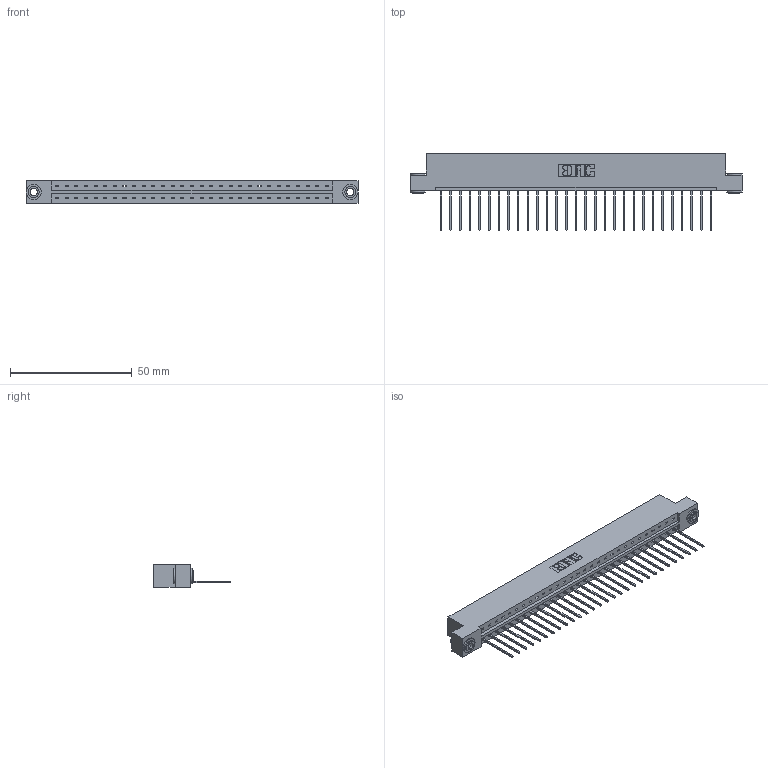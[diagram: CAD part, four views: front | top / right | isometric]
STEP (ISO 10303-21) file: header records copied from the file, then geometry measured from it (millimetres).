
FILE_DESCRIPTION (( 'STEP AP203' ), '1' );
FILE_NAME ('333-029-542-103.STEP', '2018-08-02T16:38:14', ( '' ), ( '' ), 'SwSTEP 2.0', 'SolidWorks 2016', '' );
FILE_SCHEMA (( 'CONFIG_CONTROL_DESIGN' ));
Length unit declared in the file: inch
Products named in the file (4): 333 Part_Flush - .156 Dia - TH; 345-292-001_345-293-142; 345-250-002_345-250-002-102; 333-029-542-103
Assembly tree (32 placements, depth 2):
  333-029-542-103
    333 Part_Flush - .156 Dia - TH
    345-292-001_345-293-142  x29
    345-250-002_345-250-002-102  x2
Bounding box: 136.45 x 31.63 x 9.4 mm (x, y, z)
Volume: 13702.7 mm3; surface area: 15393.5 mm2
Topology: 32 solids, 32 shells, 1834 faces, 5491 edges, 3618 vertices
Faces by surface type: plane 1298, cylinder 528, cone 8
Entity records: 20078 total; most frequent: CARTESIAN_POINT 3444, ORIENTED_EDGE 3402, DIRECTION 2965, EDGE_CURVE 1701, LINE 1549, VECTOR 1549, VERTEX_POINT 1130, AXIS2_PLACEMENT_3D 708
